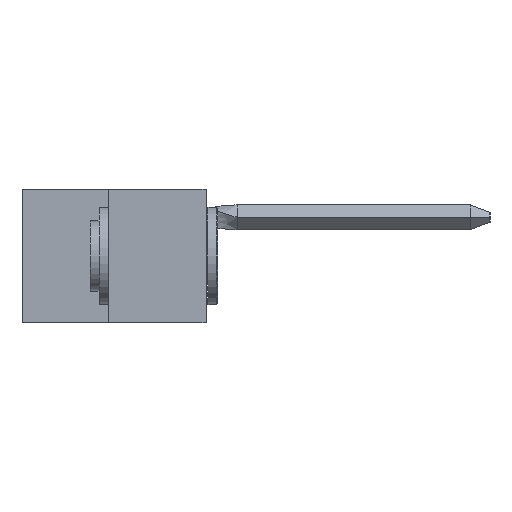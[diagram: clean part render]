
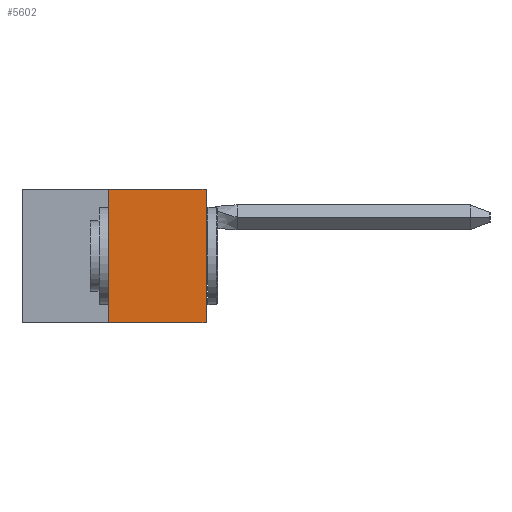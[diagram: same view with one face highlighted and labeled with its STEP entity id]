
A CAD part, left-side view. The second image highlights one B-rep face of the part: STEP entity #5602.
In plain terms, the highlighted planar face has unit normal (-1, 0, 0).
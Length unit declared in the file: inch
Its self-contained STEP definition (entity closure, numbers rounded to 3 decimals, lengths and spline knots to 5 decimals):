
#4672 = VERTEX_POINT ( 'NONE', #24486 ) ;
#5602 = ADVANCED_FACE ( 'NONE', ( #42186 ), #30021, .F. ) ;
#6208 = LINE ( 'NONE', #15367, #25201 ) ;
#9286 = ORIENTED_EDGE ( 'NONE', *, *, #24660, .T. ) ;
#11725 = EDGE_CURVE ( 'NONE', #18910, #4672, #6208, .T. ) ;
#12221 = VECTOR ( 'NONE', #39364, 39.37008 ) ;
#15367 = CARTESIAN_POINT ( 'NONE',  ( 0., 0.473, 0. ) ) ;
#17786 = CARTESIAN_POINT ( 'NONE',  ( 0., 0.473, -0.343 ) ) ;
#18910 = VERTEX_POINT ( 'NONE', #38587 ) ;
#20903 = ORIENTED_EDGE ( 'NONE', *, *, #39335, .F. ) ;
#22776 = EDGE_LOOP ( 'NONE', ( #30425, #20903, #46137, #9286 ) ) ;
#24486 = CARTESIAN_POINT ( 'NONE',  ( 0., 0., 0. ) ) ;
#24660 = EDGE_CURVE ( 'NONE', #54032, #4672, #54195, .T. ) ;
#25201 = VECTOR ( 'NONE', #37137, 39.37008 ) ;
#26990 = CARTESIAN_POINT ( 'NONE',  ( 0., 0.25, -0.343 ) ) ;
#27679 = CARTESIAN_POINT ( 'NONE',  ( 0., 0., 0. ) ) ;
#29437 = VECTOR ( 'NONE', #49379, 39.37008 ) ;
#30021 = PLANE ( 'NONE',  #34570 ) ;
#30425 = ORIENTED_EDGE ( 'NONE', *, *, #11725, .F. ) ;
#34570 = AXIS2_PLACEMENT_3D ( 'NONE', #55750, #52151, #47849 ) ;
#36383 = DIRECTION ( 'NONE',  ( 0., 0., 1. ) ) ;
#37137 = DIRECTION ( 'NONE',  ( 0., -1., 0. ) ) ;
#37242 = EDGE_CURVE ( 'NONE', #37862, #54032, #48788, .T. ) ;
#37862 = VERTEX_POINT ( 'NONE', #26990 ) ;
#38587 = CARTESIAN_POINT ( 'NONE',  ( 0., 0.25, 0. ) ) ;
#39335 = EDGE_CURVE ( 'NONE', #37862, #18910, #45019, .T. ) ;
#39364 = DIRECTION ( 'NONE',  ( 0., -1., 0. ) ) ;
#39999 = VECTOR ( 'NONE', #36383, 39.37008 ) ;
#42186 = FACE_OUTER_BOUND ( 'NONE', #22776, .T. ) ;
#45019 = LINE ( 'NONE', #45176, #29437 ) ;
#45176 = CARTESIAN_POINT ( 'NONE',  ( 0., 0.25, 0. ) ) ;
#46137 = ORIENTED_EDGE ( 'NONE', *, *, #37242, .T. ) ;
#47849 = DIRECTION ( 'NONE',  ( 0., 0., -1. ) ) ;
#48788 = LINE ( 'NONE', #17786, #12221 ) ;
#49379 = DIRECTION ( 'NONE',  ( 0., 0., 1. ) ) ;
#51692 = CARTESIAN_POINT ( 'NONE',  ( 0., 0., -0.343 ) ) ;
#52151 = DIRECTION ( 'NONE',  ( 1., 0., 0. ) ) ;
#54032 = VERTEX_POINT ( 'NONE', #51692 ) ;
#54195 = LINE ( 'NONE', #27679, #39999 ) ;
#55750 = CARTESIAN_POINT ( 'NONE',  ( 0., 0.473, 0. ) ) ;
